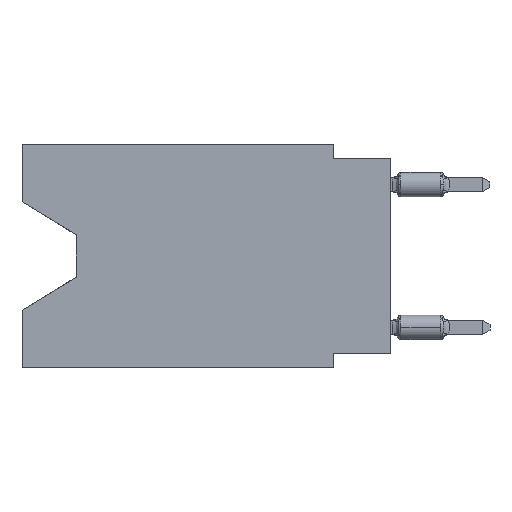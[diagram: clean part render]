
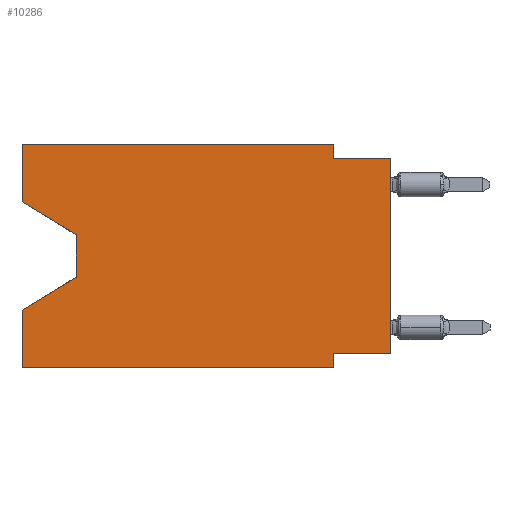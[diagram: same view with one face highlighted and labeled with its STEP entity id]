
A CAD part, left-side view. The second image highlights one B-rep face of the part: STEP entity #10286.
In plain terms, the highlighted planar face has unit normal (-1, 0, 0).
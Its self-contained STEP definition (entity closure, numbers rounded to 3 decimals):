
#157 = LINE ( 'NONE', #392, #13697 ) ;
#212 = EDGE_CURVE ( 'NONE', #7621, #5432, #14256, .T. ) ;
#352 = VECTOR ( 'NONE', #14211, 1000. ) ;
#392 = CARTESIAN_POINT ( 'NONE',  ( 0., 2.54, 0. ) ) ;
#395 = CARTESIAN_POINT ( 'NONE',  ( 0., 0., -9.271 ) ) ;
#425 = DIRECTION ( 'NONE',  ( 0., -0.855, -0.519 ) ) ;
#480 = VERTEX_POINT ( 'NONE', #1866 ) ;
#582 = LINE ( 'NONE', #7536, #12047 ) ;
#921 = VERTEX_POINT ( 'NONE', #5439 ) ;
#1240 = ORIENTED_EDGE ( 'NONE', *, *, #12059, .F. ) ;
#1486 = VERTEX_POINT ( 'NONE', #1492 ) ;
#1492 = CARTESIAN_POINT ( 'NONE',  ( 0., 16.383, -7.36 ) ) ;
#1562 = CARTESIAN_POINT ( 'NONE',  ( 0., 13.97, -4.013 ) ) ;
#1849 = LINE ( 'NONE', #6715, #2837 ) ;
#1866 = CARTESIAN_POINT ( 'NONE',  ( 0., 2.54, -9.906 ) ) ;
#1874 = ORIENTED_EDGE ( 'NONE', *, *, #5184, .F. ) ;
#2097 = VECTOR ( 'NONE', #4044, 1000. ) ;
#2101 = ORIENTED_EDGE ( 'NONE', *, *, #6119, .T. ) ;
#2126 = EDGE_CURVE ( 'NONE', #921, #7621, #1849, .T. ) ;
#2837 = VECTOR ( 'NONE', #425, 1000. ) ;
#2868 = VERTEX_POINT ( 'NONE', #12708 ) ;
#3330 = ORIENTED_EDGE ( 'NONE', *, *, #8759, .F. ) ;
#3681 = VERTEX_POINT ( 'NONE', #10549 ) ;
#3860 = EDGE_CURVE ( 'NONE', #5916, #11403, #14843, .T. ) ;
#4018 = VERTEX_POINT ( 'NONE', #15419 ) ;
#4033 = DIRECTION ( 'NONE',  ( 0., 0., 1. ) ) ;
#4038 = CARTESIAN_POINT ( 'NONE',  ( 0., 16.383, 0. ) ) ;
#4044 = DIRECTION ( 'NONE',  ( 0., 0., -1. ) ) ;
#4515 = CARTESIAN_POINT ( 'NONE',  ( 0., 13.97, -4.013 ) ) ;
#4732 = DIRECTION ( 'NONE',  ( 0., 0., -1. ) ) ;
#4867 = CARTESIAN_POINT ( 'NONE',  ( 0., 0., -9.271 ) ) ;
#4957 = ORIENTED_EDGE ( 'NONE', *, *, #7779, .F. ) ;
#5184 = EDGE_CURVE ( 'NONE', #11403, #480, #10362, .T. ) ;
#5432 = VERTEX_POINT ( 'NONE', #8500 ) ;
#5439 = CARTESIAN_POINT ( 'NONE',  ( 0., 16.383, -2.546 ) ) ;
#5658 = EDGE_CURVE ( 'NONE', #3681, #1486, #5666, .T. ) ;
#5666 = LINE ( 'NONE', #13033, #352 ) ;
#5731 = LINE ( 'NONE', #11666, #9291 ) ;
#5916 = VERTEX_POINT ( 'NONE', #395 ) ;
#6119 = EDGE_CURVE ( 'NONE', #3681, #480, #5731, .T. ) ;
#6142 = DIRECTION ( 'NONE',  ( 0., 0., 1. ) ) ;
#6173 = ORIENTED_EDGE ( 'NONE', *, *, #15453, .T. ) ;
#6715 = CARTESIAN_POINT ( 'NONE',  ( 0., 16.383, -2.546 ) ) ;
#6729 = VERTEX_POINT ( 'NONE', #4038 ) ;
#7111 = FACE_OUTER_BOUND ( 'NONE', #12841, .T. ) ;
#7417 = CARTESIAN_POINT ( 'NONE',  ( 0., 16.383, 0. ) ) ;
#7536 = CARTESIAN_POINT ( 'NONE',  ( 0., 0., -0.635 ) ) ;
#7621 = VERTEX_POINT ( 'NONE', #4515 ) ;
#7624 = CARTESIAN_POINT ( 'NONE',  ( 0., 13.97, -5.893 ) ) ;
#7776 = DIRECTION ( 'NONE',  ( 0., 0.855, -0.519 ) ) ;
#7779 = EDGE_CURVE ( 'NONE', #6729, #2868, #12596, .T. ) ;
#8181 = ORIENTED_EDGE ( 'NONE', *, *, #212, .T. ) ;
#8405 = ORIENTED_EDGE ( 'NONE', *, *, #3860, .F. ) ;
#8500 = CARTESIAN_POINT ( 'NONE',  ( 0., 13.97, -5.893 ) ) ;
#8759 = EDGE_CURVE ( 'NONE', #4018, #14812, #582, .T. ) ;
#8948 = ORIENTED_EDGE ( 'NONE', *, *, #10810, .F. ) ;
#9291 = VECTOR ( 'NONE', #15638, 1000. ) ;
#9944 = AXIS2_PLACEMENT_3D ( 'NONE', #13439, #12182, #4732 ) ;
#9976 = VECTOR ( 'NONE', #11697, 1000. ) ;
#10286 = ADVANCED_FACE ( 'NONE', ( #7111 ), #12096, .F. ) ;
#10362 = LINE ( 'NONE', #14020, #13654 ) ;
#10419 = LINE ( 'NONE', #13856, #15475 ) ;
#10549 = CARTESIAN_POINT ( 'NONE',  ( 0., 16.383, -9.906 ) ) ;
#10810 = EDGE_CURVE ( 'NONE', #2868, #4018, #157, .T. ) ;
#11161 = EDGE_CURVE ( 'NONE', #5916, #14812, #10419, .T. ) ;
#11198 = VECTOR ( 'NONE', #6142, 1000. ) ;
#11403 = VERTEX_POINT ( 'NONE', #14149 ) ;
#11620 = CARTESIAN_POINT ( 'NONE',  ( 0., 16.383, 0. ) ) ;
#11662 = VECTOR ( 'NONE', #7776, 1000. ) ;
#11666 = CARTESIAN_POINT ( 'NONE',  ( 0., 16.383, -9.906 ) ) ;
#11697 = DIRECTION ( 'NONE',  ( 0., -1., 0. ) ) ;
#11795 = DIRECTION ( 'NONE',  ( 0., 0., -1. ) ) ;
#12047 = VECTOR ( 'NONE', #13919, 1000. ) ;
#12059 = EDGE_CURVE ( 'NONE', #921, #6729, #15725, .T. ) ;
#12096 = PLANE ( 'NONE',  #9944 ) ;
#12137 = VECTOR ( 'NONE', #13419, 1000. ) ;
#12182 = DIRECTION ( 'NONE',  ( 1., 0., 0. ) ) ;
#12321 = ORIENTED_EDGE ( 'NONE', *, *, #11161, .T. ) ;
#12596 = LINE ( 'NONE', #11620, #9976 ) ;
#12708 = CARTESIAN_POINT ( 'NONE',  ( 0., 2.54, 0. ) ) ;
#12747 = LINE ( 'NONE', #7624, #11662 ) ;
#12841 = EDGE_LOOP ( 'NONE', ( #13955, #8181, #6173, #14103, #2101, #1874, #8405, #12321, #3330, #8948, #4957, #1240 ) ) ;
#13033 = CARTESIAN_POINT ( 'NONE',  ( 0., 16.383, 0. ) ) ;
#13180 = CARTESIAN_POINT ( 'NONE',  ( 0., 0., -0.635 ) ) ;
#13419 = DIRECTION ( 'NONE',  ( 0., 1., 0. ) ) ;
#13439 = CARTESIAN_POINT ( 'NONE',  ( 0., 16.383, 0. ) ) ;
#13654 = VECTOR ( 'NONE', #11795, 1000. ) ;
#13697 = VECTOR ( 'NONE', #14844, 1000. ) ;
#13856 = CARTESIAN_POINT ( 'NONE',  ( 0., 0., 0. ) ) ;
#13919 = DIRECTION ( 'NONE',  ( 0., -1., 0. ) ) ;
#13955 = ORIENTED_EDGE ( 'NONE', *, *, #2126, .T. ) ;
#14020 = CARTESIAN_POINT ( 'NONE',  ( 0., 2.54, -9.906 ) ) ;
#14103 = ORIENTED_EDGE ( 'NONE', *, *, #5658, .F. ) ;
#14149 = CARTESIAN_POINT ( 'NONE',  ( 0., 2.54, -9.271 ) ) ;
#14211 = DIRECTION ( 'NONE',  ( 0., 0., 1. ) ) ;
#14256 = LINE ( 'NONE', #1562, #2097 ) ;
#14812 = VERTEX_POINT ( 'NONE', #13180 ) ;
#14843 = LINE ( 'NONE', #4867, #12137 ) ;
#14844 = DIRECTION ( 'NONE',  ( 0., 0., -1. ) ) ;
#15419 = CARTESIAN_POINT ( 'NONE',  ( 0., 2.54, -0.635 ) ) ;
#15453 = EDGE_CURVE ( 'NONE', #5432, #1486, #12747, .T. ) ;
#15475 = VECTOR ( 'NONE', #4033, 1000. ) ;
#15638 = DIRECTION ( 'NONE',  ( 0., -1., 0. ) ) ;
#15725 = LINE ( 'NONE', #7417, #11198 ) ;
